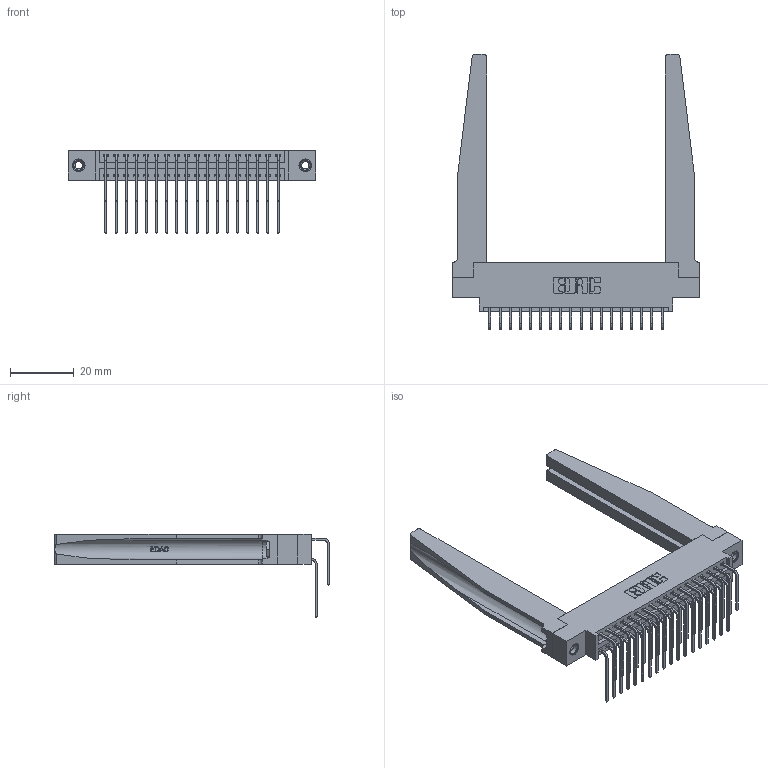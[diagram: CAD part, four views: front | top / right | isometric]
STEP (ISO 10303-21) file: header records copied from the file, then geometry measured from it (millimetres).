
FILE_DESCRIPTION (( 'STEP AP203' ), '1' );
FILE_NAME ('346-036-559-878.STEP', '2022-05-19T22:34:55', ( '' ), ( '' ), 'SwSTEP 2.0', 'SolidWorks 2020', '' );
FILE_SCHEMA (( 'CONFIG_CONTROL_DESIGN' ));
Length unit declared in the file: inch
Products named in the file (6): 345-292-001_559 Tail - 2; 346-220-078_345-220-078; 345-250-001_345-250-001-102; 346 Part_0.170 Offset - 0.156 Dia-TH; 345-292-001_558 559 Tail - 1; 346-036-559-878
Assembly tree (41 placements, depth 2):
  346-036-559-878
    346 Part_0.170 Offset - 0.156 Dia-TH
    345-292-001_558 559 Tail - 1  x18
    345-292-001_559 Tail - 2  x18
    346-220-078_345-220-078  x2
    345-250-001_345-250-001-102  x2
Bounding box: 77.72 x 86.17 x 26.16 mm (x, y, z)
Volume: 14336.5 mm3; surface area: 17580.5 mm2
Topology: 41 solids, 41 shells, 2318 faces, 6781 edges, 4462 vertices
Faces by surface type: plane 1568, cylinder 698, bspline 36, cone 12, torus 4
Entity records: 22058 total; most frequent: CARTESIAN_POINT 4664, ORIENTED_EDGE 3434, DIRECTION 3119, EDGE_CURVE 1717, VECTOR 1379, LINE 1379, VERTEX_POINT 1136, AXIS2_PLACEMENT_3D 870
